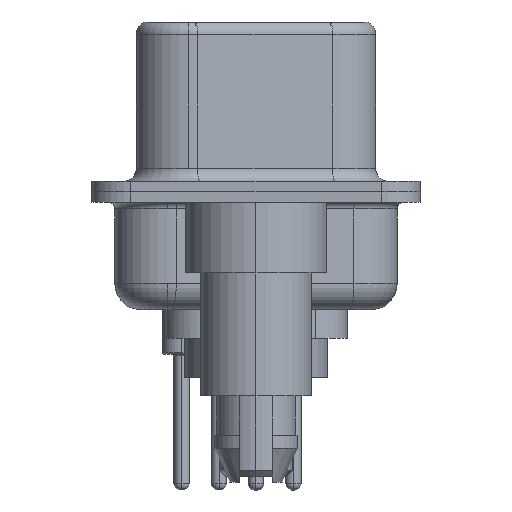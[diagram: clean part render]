
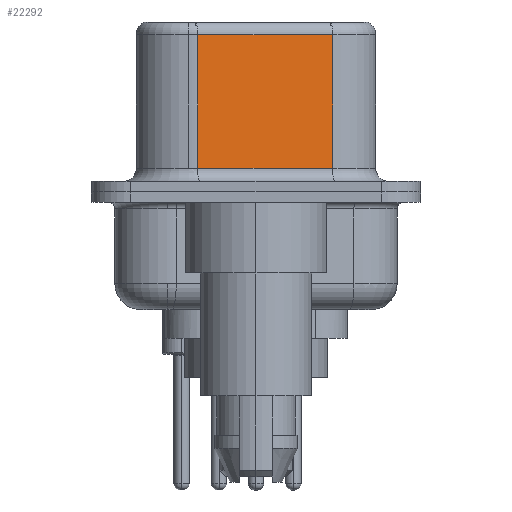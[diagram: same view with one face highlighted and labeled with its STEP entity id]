
A CAD part, left-side view. The second image highlights one B-rep face of the part: STEP entity #22292.
In plain terms, the highlighted planar face has unit normal (-0.985, -0.174, 0).
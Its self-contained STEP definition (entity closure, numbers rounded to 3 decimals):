
#764 = DIRECTION ( 'NONE',  ( 0., 0., -1. ) ) ;
#1157 = VECTOR ( 'NONE', #764, 1000. ) ;
#2554 = CARTESIAN_POINT ( 'NONE',  ( 4.58, -2.927, 6.52 ) ) ;
#2907 = CARTESIAN_POINT ( 'NONE',  ( 4.58, -2.927, 6.52 ) ) ;
#2982 = LINE ( 'NONE', #23233, #25031 ) ;
#3158 = FACE_OUTER_BOUND ( 'NONE', #23318, .T. ) ;
#4880 = CARTESIAN_POINT ( 'NONE',  ( 3.67, 2.233, 6.52 ) ) ;
#7363 = EDGE_CURVE ( 'NONE', #16565, #21461, #2982, .T. ) ;
#9873 = EDGE_CURVE ( 'NONE', #12808, #16565, #12544, .T. ) ;
#10536 = CARTESIAN_POINT ( 'NONE',  ( 4.58, -2.927, 6.02 ) ) ;
#11039 = DIRECTION ( 'NONE',  ( -0.174, 0.985, 0. ) ) ;
#12358 = CARTESIAN_POINT ( 'NONE',  ( 3.67, 2.233, 0.9 ) ) ;
#12405 = LINE ( 'NONE', #2907, #1157 ) ;
#12544 = LINE ( 'NONE', #4880, #17591 ) ;
#12808 = VERTEX_POINT ( 'NONE', #27205 ) ;
#15444 = DIRECTION ( 'NONE',  ( 0., 0., -1. ) ) ;
#15962 = CARTESIAN_POINT ( 'NONE',  ( 4.58, -2.927, 0.9 ) ) ;
#16565 = VERTEX_POINT ( 'NONE', #12358 ) ;
#16787 = DIRECTION ( 'NONE',  ( 0.174, -0.985, 0. ) ) ;
#17044 = ORIENTED_EDGE ( 'NONE', *, *, #7363, .T. ) ;
#17294 = AXIS2_PLACEMENT_3D ( 'NONE', #2554, #23928, #11039 ) ;
#17509 = ORIENTED_EDGE ( 'NONE', *, *, #9873, .T. ) ;
#17591 = VECTOR ( 'NONE', #15444, 1000. ) ;
#18647 = CARTESIAN_POINT ( 'NONE',  ( 4.58, -2.927, 6.02 ) ) ;
#20427 = VECTOR ( 'NONE', #23436, 1000. ) ;
#20668 = ORIENTED_EDGE ( 'NONE', *, *, #22409, .F. ) ;
#21089 = LINE ( 'NONE', #10536, #20427 ) ;
#21461 = VERTEX_POINT ( 'NONE', #15962 ) ;
#21780 = PLANE ( 'NONE',  #17294 ) ;
#22292 = ADVANCED_FACE ( 'NONE', ( #3158 ), #21780, .F. ) ;
#22409 = EDGE_CURVE ( 'NONE', #26204, #21461, #12405, .T. ) ;
#23216 = ORIENTED_EDGE ( 'NONE', *, *, #23942, .T. ) ;
#23233 = CARTESIAN_POINT ( 'NONE',  ( 4.58, -2.927, 0.9 ) ) ;
#23318 = EDGE_LOOP ( 'NONE', ( #20668, #23216, #17509, #17044 ) ) ;
#23436 = DIRECTION ( 'NONE',  ( -0.174, 0.985, 0. ) ) ;
#23928 = DIRECTION ( 'NONE',  ( 0.985, 0.174, 0. ) ) ;
#23942 = EDGE_CURVE ( 'NONE', #26204, #12808, #21089, .T. ) ;
#25031 = VECTOR ( 'NONE', #16787, 1000. ) ;
#26204 = VERTEX_POINT ( 'NONE', #18647 ) ;
#27205 = CARTESIAN_POINT ( 'NONE',  ( 3.67, 2.233, 6.02 ) ) ;
